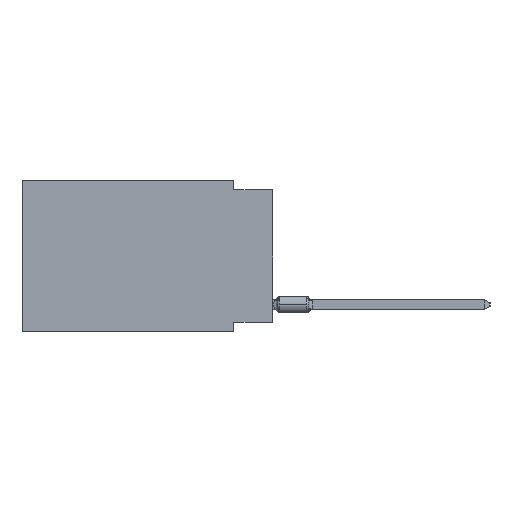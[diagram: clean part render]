
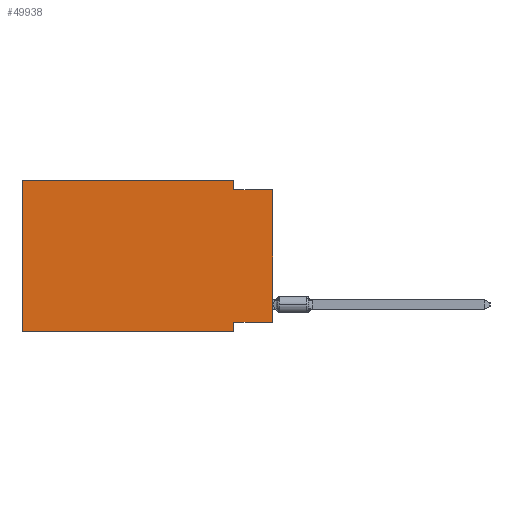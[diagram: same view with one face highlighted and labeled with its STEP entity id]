
A CAD part, left-side view. The second image highlights one B-rep face of the part: STEP entity #49938.
In plain terms, the highlighted planar face has unit normal (-1, 0, 0).
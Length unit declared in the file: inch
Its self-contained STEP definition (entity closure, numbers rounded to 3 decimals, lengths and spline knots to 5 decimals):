
#1450 = EDGE_CURVE ( 'NONE', #50702, #65901, #70566, .T. ) ;
#2166 = AXIS2_PLACEMENT_3D ( 'NONE', #34171, #28005, #39248 ) ;
#3722 = ORIENTED_EDGE ( 'NONE', *, *, #5358, .T. ) ;
#4308 = LINE ( 'NONE', #58002, #52683 ) ;
#4525 = CARTESIAN_POINT ( 'NONE',  ( 0., 0., -0.025 ) ) ;
#5358 = EDGE_CURVE ( 'NONE', #17044, #65453, #15948, .T. ) ;
#6570 = CARTESIAN_POINT ( 'NONE',  ( 0., 0.1, -0.39 ) ) ;
#9081 = EDGE_CURVE ( 'NONE', #33026, #14746, #26205, .T. ) ;
#10042 = CARTESIAN_POINT ( 'NONE',  ( 0., 0.645, -0.39 ) ) ;
#10316 = DIRECTION ( 'NONE',  ( 0., -1., 0. ) ) ;
#13534 = CARTESIAN_POINT ( 'NONE',  ( 0., 0.645, 0. ) ) ;
#14746 = VERTEX_POINT ( 'NONE', #39045 ) ;
#15948 = LINE ( 'NONE', #21055, #42755 ) ;
#17044 = VERTEX_POINT ( 'NONE', #28509 ) ;
#17330 = EDGE_LOOP ( 'NONE', ( #3722, #69021, #68219, #69216, #53156, #53150, #26407, #68901 ) ) ;
#20867 = LINE ( 'NONE', #4525, #65493 ) ;
#21055 = CARTESIAN_POINT ( 'NONE',  ( 0., 0., 0. ) ) ;
#22481 = LINE ( 'NONE', #39870, #28860 ) ;
#22760 = CARTESIAN_POINT ( 'NONE',  ( 0., 0.1, 0. ) ) ;
#24451 = CARTESIAN_POINT ( 'NONE',  ( 0., 0., -0.365 ) ) ;
#25272 = EDGE_CURVE ( 'NONE', #17044, #65990, #51647, .T. ) ;
#25562 = CARTESIAN_POINT ( 'NONE',  ( 0., 0., -0.025 ) ) ;
#26182 = EDGE_CURVE ( 'NONE', #33026, #40222, #4308, .T. ) ;
#26205 = LINE ( 'NONE', #49407, #50323 ) ;
#26407 = ORIENTED_EDGE ( 'NONE', *, *, #50313, .F. ) ;
#28005 = DIRECTION ( 'NONE',  ( 1., 0., 0. ) ) ;
#28419 = EDGE_CURVE ( 'NONE', #14746, #50702, #46533, .T. ) ;
#28509 = CARTESIAN_POINT ( 'NONE',  ( 0., 0., -0.365 ) ) ;
#28860 = VECTOR ( 'NONE', #44969, 39.37008 ) ;
#31787 = CARTESIAN_POINT ( 'NONE',  ( 0., 0.1, 0. ) ) ;
#33026 = VERTEX_POINT ( 'NONE', #10042 ) ;
#34171 = CARTESIAN_POINT ( 'NONE',  ( 0., 0.645, 0. ) ) ;
#39045 = CARTESIAN_POINT ( 'NONE',  ( 0., 0.645, 0. ) ) ;
#39248 = DIRECTION ( 'NONE',  ( 0., 0., -1. ) ) ;
#39870 = CARTESIAN_POINT ( 'NONE',  ( 0., 0.1, -0.39 ) ) ;
#40222 = VERTEX_POINT ( 'NONE', #6570 ) ;
#41673 = DIRECTION ( 'NONE',  ( 0., -1., 0. ) ) ;
#42755 = VECTOR ( 'NONE', #66335, 39.37008 ) ;
#44969 = DIRECTION ( 'NONE',  ( 0., 0., -1. ) ) ;
#45626 = VECTOR ( 'NONE', #47745, 39.37008 ) ;
#46188 = DIRECTION ( 'NONE',  ( 0., -1., 0. ) ) ;
#46533 = LINE ( 'NONE', #13534, #57395 ) ;
#47745 = DIRECTION ( 'NONE',  ( 0., 0., -1. ) ) ;
#48952 = CARTESIAN_POINT ( 'NONE',  ( 0., 0.1, -0.025 ) ) ;
#49407 = CARTESIAN_POINT ( 'NONE',  ( 0., 0.645, 0. ) ) ;
#49938 = ADVANCED_FACE ( 'NONE', ( #60305 ), #54860, .F. ) ;
#50313 = EDGE_CURVE ( 'NONE', #65990, #40222, #22481, .T. ) ;
#50323 = VECTOR ( 'NONE', #71135, 39.37008 ) ;
#50702 = VERTEX_POINT ( 'NONE', #22760 ) ;
#51085 = CARTESIAN_POINT ( 'NONE',  ( 0., 0.1, -0.365 ) ) ;
#51647 = LINE ( 'NONE', #24451, #54925 ) ;
#52683 = VECTOR ( 'NONE', #41673, 39.37008 ) ;
#53150 = ORIENTED_EDGE ( 'NONE', *, *, #26182, .T. ) ;
#53156 = ORIENTED_EDGE ( 'NONE', *, *, #9081, .F. ) ;
#54860 = PLANE ( 'NONE',  #2166 ) ;
#54925 = VECTOR ( 'NONE', #67969, 39.37008 ) ;
#57395 = VECTOR ( 'NONE', #46188, 39.37008 ) ;
#58002 = CARTESIAN_POINT ( 'NONE',  ( 0., 0.645, -0.39 ) ) ;
#60305 = FACE_OUTER_BOUND ( 'NONE', #17330, .T. ) ;
#65439 = EDGE_CURVE ( 'NONE', #65901, #65453, #20867, .T. ) ;
#65453 = VERTEX_POINT ( 'NONE', #25562 ) ;
#65493 = VECTOR ( 'NONE', #10316, 39.37008 ) ;
#65901 = VERTEX_POINT ( 'NONE', #48952 ) ;
#65990 = VERTEX_POINT ( 'NONE', #51085 ) ;
#66335 = DIRECTION ( 'NONE',  ( 0., 0., 1. ) ) ;
#67969 = DIRECTION ( 'NONE',  ( 0., 1., 0. ) ) ;
#68219 = ORIENTED_EDGE ( 'NONE', *, *, #1450, .F. ) ;
#68901 = ORIENTED_EDGE ( 'NONE', *, *, #25272, .F. ) ;
#69021 = ORIENTED_EDGE ( 'NONE', *, *, #65439, .F. ) ;
#69216 = ORIENTED_EDGE ( 'NONE', *, *, #28419, .F. ) ;
#70566 = LINE ( 'NONE', #31787, #45626 ) ;
#71135 = DIRECTION ( 'NONE',  ( 0., 0., 1. ) ) ;
